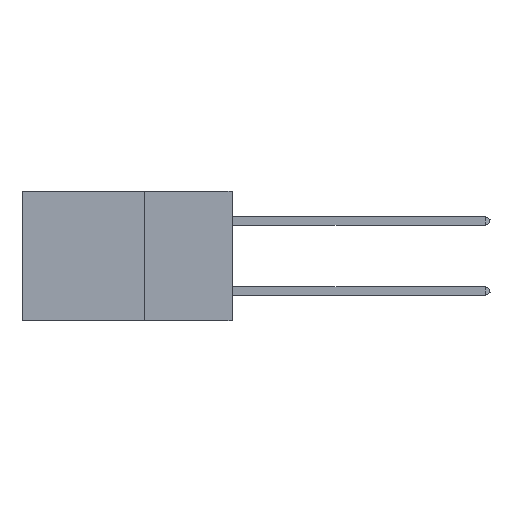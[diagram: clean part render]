
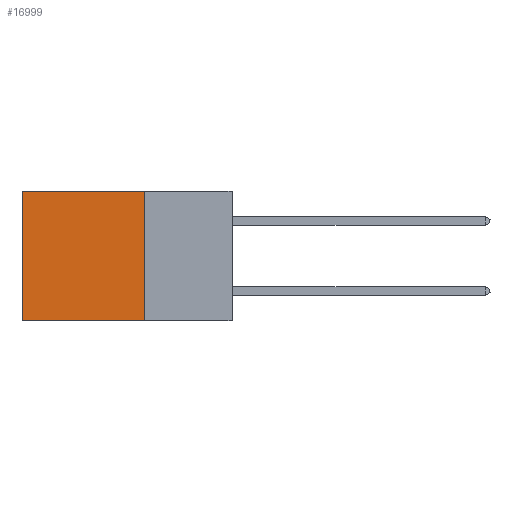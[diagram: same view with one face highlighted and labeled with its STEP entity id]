
A CAD part, left-side view. The second image highlights one B-rep face of the part: STEP entity #16999.
In plain terms, the highlighted planar face has unit normal (-1, 0, 0).
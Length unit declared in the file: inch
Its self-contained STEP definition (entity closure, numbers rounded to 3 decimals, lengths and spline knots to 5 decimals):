
#1038 = VERTEX_POINT ( 'NONE', #13133 ) ;
#1389 = DIRECTION ( 'NONE',  ( 0., 1., 0. ) ) ;
#2891 = CARTESIAN_POINT ( 'NONE',  ( 0.2875, 0.6, 0. ) ) ;
#4093 = VECTOR ( 'NONE', #1389, 39.37008 ) ;
#5436 = CARTESIAN_POINT ( 'NONE',  ( 0.2875, 0.25, 0. ) ) ;
#5974 = VERTEX_POINT ( 'NONE', #24249 ) ;
#5982 = CARTESIAN_POINT ( 'NONE',  ( 0.2875, 0.25, 0. ) ) ;
#6207 = VERTEX_POINT ( 'NONE', #2891 ) ;
#6282 = VECTOR ( 'NONE', #15623, 39.37008 ) ;
#7130 = CARTESIAN_POINT ( 'NONE',  ( 0.2875, 0.25, 0. ) ) ;
#7299 = VECTOR ( 'NONE', #23085, 39.37008 ) ;
#9317 = EDGE_CURVE ( 'NONE', #22881, #6207, #25584, .T. ) ;
#10014 = ORIENTED_EDGE ( 'NONE', *, *, #31044, .F. ) ;
#11162 = EDGE_CURVE ( 'NONE', #6207, #5974, #26209, .T. ) ;
#13054 = CARTESIAN_POINT ( 'NONE',  ( 0.2875, 0.6, 0. ) ) ;
#13133 = CARTESIAN_POINT ( 'NONE',  ( 0.2875, 0.25, -0.37 ) ) ;
#13448 = LINE ( 'NONE', #7130, #24753 ) ;
#14011 = PLANE ( 'NONE',  #22773 ) ;
#15623 = DIRECTION ( 'NONE',  ( 0., 1., 0. ) ) ;
#15711 = EDGE_LOOP ( 'NONE', ( #16118, #10014, #24848, #22266 ) ) ;
#16118 = ORIENTED_EDGE ( 'NONE', *, *, #11162, .T. ) ;
#16999 = ADVANCED_FACE ( 'NONE', ( #28033 ), #14011, .F. ) ;
#17335 = LINE ( 'NONE', #21063, #4093 ) ;
#20627 = EDGE_CURVE ( 'NONE', #22881, #1038, #13448, .T. ) ;
#20873 = CARTESIAN_POINT ( 'NONE',  ( 0.2875, 0.25, 0. ) ) ;
#21063 = CARTESIAN_POINT ( 'NONE',  ( 0.2875, 0.25, -0.37 ) ) ;
#21807 = DIRECTION ( 'NONE',  ( 0., 0., -1. ) ) ;
#22266 = ORIENTED_EDGE ( 'NONE', *, *, #9317, .T. ) ;
#22773 = AXIS2_PLACEMENT_3D ( 'NONE', #20873, #25949, #23622 ) ;
#22881 = VERTEX_POINT ( 'NONE', #5436 ) ;
#23085 = DIRECTION ( 'NONE',  ( 0., 0., -1. ) ) ;
#23622 = DIRECTION ( 'NONE',  ( 0., 0., -1. ) ) ;
#24249 = CARTESIAN_POINT ( 'NONE',  ( 0.2875, 0.6, -0.37 ) ) ;
#24753 = VECTOR ( 'NONE', #21807, 39.37008 ) ;
#24848 = ORIENTED_EDGE ( 'NONE', *, *, #20627, .F. ) ;
#25584 = LINE ( 'NONE', #5982, #6282 ) ;
#25949 = DIRECTION ( 'NONE',  ( 1., 0., 0. ) ) ;
#26209 = LINE ( 'NONE', #13054, #7299 ) ;
#28033 = FACE_OUTER_BOUND ( 'NONE', #15711, .T. ) ;
#31044 = EDGE_CURVE ( 'NONE', #1038, #5974, #17335, .T. ) ;
